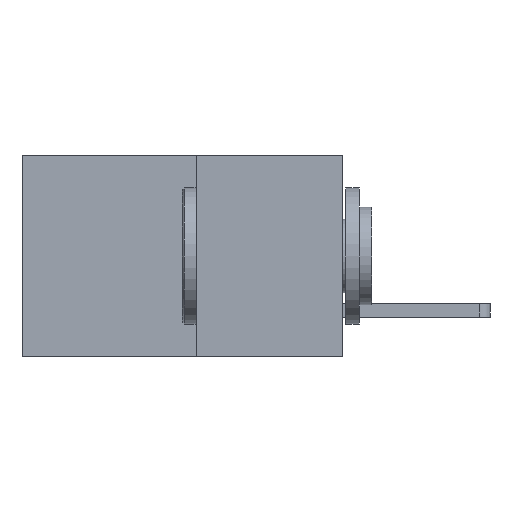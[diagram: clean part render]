
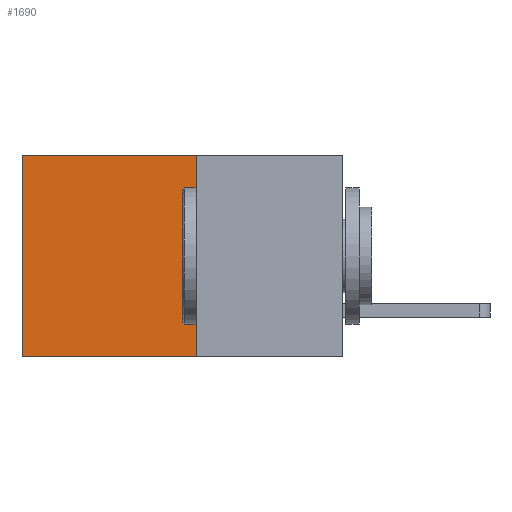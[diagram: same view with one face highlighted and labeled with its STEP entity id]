
A CAD part, left-side view. The second image highlights one B-rep face of the part: STEP entity #1690.
In plain terms, the highlighted planar face has unit normal (-1, 0, 0).
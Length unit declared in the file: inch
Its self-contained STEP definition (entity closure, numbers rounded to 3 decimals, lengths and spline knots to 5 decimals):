
#229 = ORIENTED_EDGE ( 'NONE', *, *, #8498, .T. ) ;
#982 = VERTEX_POINT ( 'NONE', #6456 ) ;
#1404 = VERTEX_POINT ( 'NONE', #3439 ) ;
#1427 = DIRECTION ( 'NONE',  ( 0., 1., 0. ) ) ;
#1690 = ADVANCED_FACE ( 'NONE', ( #2694 ), #4754, .F. ) ;
#2298 = VECTOR ( 'NONE', #6802, 39.37008 ) ;
#2694 = FACE_OUTER_BOUND ( 'NONE', #3399, .T. ) ;
#2730 = VECTOR ( 'NONE', #1427, 39.37008 ) ;
#3235 = CARTESIAN_POINT ( 'NONE',  ( 0.277, 0.59, -0.37 ) ) ;
#3344 = LINE ( 'NONE', #3235, #8516 ) ;
#3399 = EDGE_LOOP ( 'NONE', ( #8197, #3892, #4652, #229 ) ) ;
#3439 = CARTESIAN_POINT ( 'NONE',  ( 0.277, 0.59, 0. ) ) ;
#3892 = ORIENTED_EDGE ( 'NONE', *, *, #5539, .F. ) ;
#4090 = LINE ( 'NONE', #8126, #2298 ) ;
#4192 = CARTESIAN_POINT ( 'NONE',  ( 0.277, 0.27, -0.37 ) ) ;
#4271 = CARTESIAN_POINT ( 'NONE',  ( 0.277, 0.27, 0. ) ) ;
#4419 = LINE ( 'NONE', #8480, #8002 ) ;
#4456 = VERTEX_POINT ( 'NONE', #8261 ) ;
#4652 = ORIENTED_EDGE ( 'NONE', *, *, #8288, .F. ) ;
#4754 = PLANE ( 'NONE',  #5383 ) ;
#4846 = DIRECTION ( 'NONE',  ( 1., 0., 0. ) ) ;
#5383 = AXIS2_PLACEMENT_3D ( 'NONE', #6171, #4846, #7083 ) ;
#5539 = EDGE_CURVE ( 'NONE', #4456, #982, #6524, .T. ) ;
#5782 = DIRECTION ( 'NONE',  ( 0., 1., 0. ) ) ;
#5959 = DIRECTION ( 'NONE',  ( 0., 0., -1. ) ) ;
#6171 = CARTESIAN_POINT ( 'NONE',  ( 0.277, 0.27, -0.37 ) ) ;
#6451 = VERTEX_POINT ( 'NONE', #4271 ) ;
#6456 = CARTESIAN_POINT ( 'NONE',  ( 0.277, 0.59, -0.37 ) ) ;
#6524 = LINE ( 'NONE', #4192, #2730 ) ;
#6802 = DIRECTION ( 'NONE',  ( 0., 0., -1. ) ) ;
#7083 = DIRECTION ( 'NONE',  ( 0., 0., -1. ) ) ;
#8002 = VECTOR ( 'NONE', #5782, 39.37008 ) ;
#8126 = CARTESIAN_POINT ( 'NONE',  ( 0.277, 0.27, -0.37 ) ) ;
#8197 = ORIENTED_EDGE ( 'NONE', *, *, #8640, .T. ) ;
#8261 = CARTESIAN_POINT ( 'NONE',  ( 0.277, 0.27, -0.37 ) ) ;
#8288 = EDGE_CURVE ( 'NONE', #6451, #4456, #4090, .T. ) ;
#8480 = CARTESIAN_POINT ( 'NONE',  ( 0.277, 0.27, 0. ) ) ;
#8498 = EDGE_CURVE ( 'NONE', #6451, #1404, #4419, .T. ) ;
#8516 = VECTOR ( 'NONE', #5959, 39.37008 ) ;
#8640 = EDGE_CURVE ( 'NONE', #1404, #982, #3344, .T. ) ;
